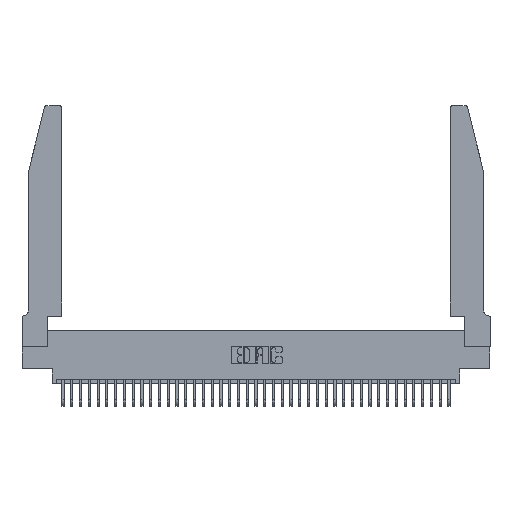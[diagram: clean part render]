
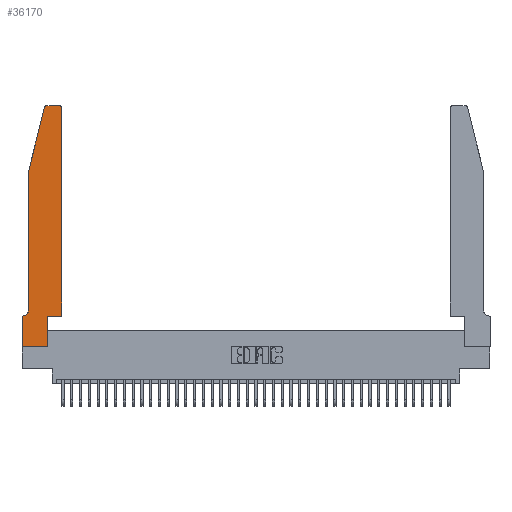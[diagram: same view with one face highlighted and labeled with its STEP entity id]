
A CAD part, top view. The second image highlights one B-rep face of the part: STEP entity #36170.
In plain terms, the highlighted planar face has unit normal (0, 0, 1).
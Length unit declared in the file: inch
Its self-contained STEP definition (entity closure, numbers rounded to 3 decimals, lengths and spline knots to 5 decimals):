
#39 = EDGE_CURVE ( 'NONE', #26336, #33545, #32935, .T. ) ;
#330 = DIRECTION ( 'NONE',  ( 1., 0., 0. ) ) ;
#1703 = DIRECTION ( 'NONE',  ( 1., 0., 0. ) ) ;
#1764 = ORIENTED_EDGE ( 'NONE', *, *, #22997, .T. ) ;
#2134 = VECTOR ( 'NONE', #20769, 39.37008 ) ;
#2223 = DIRECTION ( 'NONE',  ( 1., 0., 0. ) ) ;
#2799 = VERTEX_POINT ( 'NONE', #5036 ) ;
#3529 = DIRECTION ( 'NONE',  ( 0., -1., 0. ) ) ;
#3558 = CARTESIAN_POINT ( 'NONE',  ( 0.25487, 2.72718, 0.37 ) ) ;
#4007 = DIRECTION ( 'NONE',  ( 0., 0., -1. ) ) ;
#5036 = CARTESIAN_POINT ( 'NONE',  ( 0.4205, 2.75, 0.37 ) ) ;
#6354 = CARTESIAN_POINT ( 'NONE',  ( 0.4505, 0.35, 0.37 ) ) ;
#6504 = DIRECTION ( 'NONE',  ( 0., 0., 1. ) ) ;
#7544 = LINE ( 'NONE', #40903, #23651 ) ;
#7611 = CARTESIAN_POINT ( 'NONE',  ( 0.2865, 0., 0.37 ) ) ;
#8008 = ORIENTED_EDGE ( 'NONE', *, *, #18625, .T. ) ;
#8134 = LINE ( 'NONE', #36217, #24242 ) ;
#9564 = EDGE_CURVE ( 'NONE', #28459, #26336, #32304, .T. ) ;
#9852 = VECTOR ( 'NONE', #1703, 39.37008 ) ;
#10483 = VECTOR ( 'NONE', #25124, 39.37008 ) ;
#10577 = ORIENTED_EDGE ( 'NONE', *, *, #33723, .T. ) ;
#10963 = AXIS2_PLACEMENT_3D ( 'NONE', #40555, #21464, #2223 ) ;
#11001 = CARTESIAN_POINT ( 'NONE',  ( 0.0755, 0.42, 0.37 ) ) ;
#11203 = EDGE_CURVE ( 'NONE', #27069, #28459, #7544, .T. ) ;
#11413 = EDGE_CURVE ( 'NONE', #17808, #34038, #26142, .T. ) ;
#11830 = VERTEX_POINT ( 'NONE', #27805 ) ;
#14156 = ORIENTED_EDGE ( 'NONE', *, *, #41145, .T. ) ;
#14721 = ORIENTED_EDGE ( 'NONE', *, *, #9564, .T. ) ;
#15396 = CARTESIAN_POINT ( 'NONE',  ( 0.4205, 2.72, 0.37 ) ) ;
#15744 = CIRCLE ( 'NONE', #22930, 0.03 ) ;
#16608 = CARTESIAN_POINT ( 'NONE',  ( 0.2605, 2.75, 0.37 ) ) ;
#17002 = DIRECTION ( 'NONE',  ( -1., 0., 0. ) ) ;
#17808 = VERTEX_POINT ( 'NONE', #19049 ) ;
#17865 = EDGE_LOOP ( 'NONE', ( #38993, #36981, #41061, #28890, #14156, #8008, #31757, #14721, #25456, #1764, #19545, #10577 ) ) ;
#18078 = DIRECTION ( 'NONE',  ( 0., 1., 0. ) ) ;
#18625 = EDGE_CURVE ( 'NONE', #35926, #27069, #8134, .T. ) ;
#18635 = DIRECTION ( 'NONE',  ( 1., 0., 0. ) ) ;
#18650 = CARTESIAN_POINT ( 'NONE',  ( 0.0755, 2., 0.37 ) ) ;
#19049 = CARTESIAN_POINT ( 'NONE',  ( 0.0755, 2., 0.37 ) ) ;
#19533 = CARTESIAN_POINT ( 'NONE',  ( 0.0755, 2., 0.37 ) ) ;
#19545 = ORIENTED_EDGE ( 'NONE', *, *, #27048, .T. ) ;
#19844 = DIRECTION ( 'NONE',  ( -1., 0., 0. ) ) ;
#20769 = DIRECTION ( 'NONE',  ( 0., 1., 0. ) ) ;
#21366 = EDGE_CURVE ( 'NONE', #22048, #17808, #28584, .T. ) ;
#21464 = DIRECTION ( 'NONE',  ( 0., 0., 1. ) ) ;
#22048 = VERTEX_POINT ( 'NONE', #3558 ) ;
#22567 = VERTEX_POINT ( 'NONE', #6354 ) ;
#22857 = CARTESIAN_POINT ( 'NONE',  ( 0., 0., 0.37 ) ) ;
#22930 = AXIS2_PLACEMENT_3D ( 'NONE', #15396, #37802, #18635 ) ;
#22997 = EDGE_CURVE ( 'NONE', #33545, #22567, #26932, .T. ) ;
#23254 = CARTESIAN_POINT ( 'NONE',  ( 0.0055, 0.42, 0.37 ) ) ;
#23651 = VECTOR ( 'NONE', #28131, 39.37008 ) ;
#23783 = AXIS2_PLACEMENT_3D ( 'NONE', #31501, #6504, #28949 ) ;
#24014 = CARTESIAN_POINT ( 'NONE',  ( 0., 0.35, 0.37 ) ) ;
#24134 = LINE ( 'NONE', #16608, #31657 ) ;
#24242 = VECTOR ( 'NONE', #17002, 39.37008 ) ;
#25124 = DIRECTION ( 'NONE',  ( -0.239, -0.971, 0. ) ) ;
#25161 = FACE_OUTER_BOUND ( 'NONE', #17865, .T. ) ;
#25456 = ORIENTED_EDGE ( 'NONE', *, *, #39, .T. ) ;
#25618 = VERTEX_POINT ( 'NONE', #33072 ) ;
#26142 = LINE ( 'NONE', #19533, #41059 ) ;
#26336 = VERTEX_POINT ( 'NONE', #7611 ) ;
#26471 = DIRECTION ( 'NONE',  ( -1., 0., 0. ) ) ;
#26932 = LINE ( 'NONE', #37029, #9852 ) ;
#27048 = EDGE_CURVE ( 'NONE', #22567, #11830, #37254, .T. ) ;
#27069 = VERTEX_POINT ( 'NONE', #24014 ) ;
#27083 = CARTESIAN_POINT ( 'NONE',  ( 0.4505, 0.35, 0.37 ) ) ;
#27805 = CARTESIAN_POINT ( 'NONE',  ( 0.4505, 2.72, 0.37 ) ) ;
#28131 = DIRECTION ( 'NONE',  ( 0., -1., 0. ) ) ;
#28217 = AXIS2_PLACEMENT_3D ( 'NONE', #23254, #4007, #26471 ) ;
#28459 = VERTEX_POINT ( 'NONE', #34278 ) ;
#28584 = LINE ( 'NONE', #18650, #10483 ) ;
#28890 = ORIENTED_EDGE ( 'NONE', *, *, #11413, .T. ) ;
#28949 = DIRECTION ( 'NONE',  ( 1., 0., 0. ) ) ;
#29100 = EDGE_CURVE ( 'NONE', #25618, #22048, #38546, .T. ) ;
#30878 = CARTESIAN_POINT ( 'NONE',  ( 0.2865, 0.35, 0.37 ) ) ;
#31320 = VECTOR ( 'NONE', #330, 39.37008 ) ;
#31501 = CARTESIAN_POINT ( 'NONE',  ( 0., 0.35, 0.37 ) ) ;
#31657 = VECTOR ( 'NONE', #19844, 39.37008 ) ;
#31757 = ORIENTED_EDGE ( 'NONE', *, *, #11203, .T. ) ;
#32304 = LINE ( 'NONE', #22857, #31320 ) ;
#32935 = LINE ( 'NONE', #30878, #40355 ) ;
#33072 = CARTESIAN_POINT ( 'NONE',  ( 0.284, 2.75, 0.37 ) ) ;
#33545 = VERTEX_POINT ( 'NONE', #36970 ) ;
#33723 = EDGE_CURVE ( 'NONE', #11830, #2799, #15744, .T. ) ;
#34013 = CIRCLE ( 'NONE', #28217, 0.07 ) ;
#34038 = VERTEX_POINT ( 'NONE', #11001 ) ;
#34278 = CARTESIAN_POINT ( 'NONE',  ( 0., 0., 0.37 ) ) ;
#35926 = VERTEX_POINT ( 'NONE', #39930 ) ;
#36170 = ADVANCED_FACE ( 'NONE', ( #25161 ), #40890, .T. ) ;
#36217 = CARTESIAN_POINT ( 'NONE',  ( 0.0755, 0.35, 0.37 ) ) ;
#36970 = CARTESIAN_POINT ( 'NONE',  ( 0.2865, 0.35, 0.37 ) ) ;
#36981 = ORIENTED_EDGE ( 'NONE', *, *, #29100, .T. ) ;
#37029 = CARTESIAN_POINT ( 'NONE',  ( 0.4505, 0.35, 0.37 ) ) ;
#37254 = LINE ( 'NONE', #27083, #2134 ) ;
#37802 = DIRECTION ( 'NONE',  ( 0., 0., 1. ) ) ;
#38546 = CIRCLE ( 'NONE', #10963, 0.03 ) ;
#38993 = ORIENTED_EDGE ( 'NONE', *, *, #39588, .T. ) ;
#39588 = EDGE_CURVE ( 'NONE', #2799, #25618, #24134, .T. ) ;
#39930 = CARTESIAN_POINT ( 'NONE',  ( 0.0055, 0.35, 0.37 ) ) ;
#40355 = VECTOR ( 'NONE', #18078, 39.37008 ) ;
#40555 = CARTESIAN_POINT ( 'NONE',  ( 0.284, 2.72, 0.37 ) ) ;
#40890 = PLANE ( 'NONE',  #23783 ) ;
#40903 = CARTESIAN_POINT ( 'NONE',  ( 0., 0., 0.37 ) ) ;
#41059 = VECTOR ( 'NONE', #3529, 39.37008 ) ;
#41061 = ORIENTED_EDGE ( 'NONE', *, *, #21366, .T. ) ;
#41145 = EDGE_CURVE ( 'NONE', #34038, #35926, #34013, .T. ) ;
